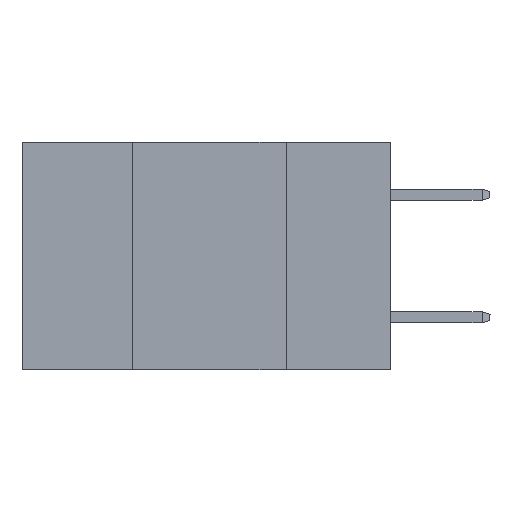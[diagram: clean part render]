
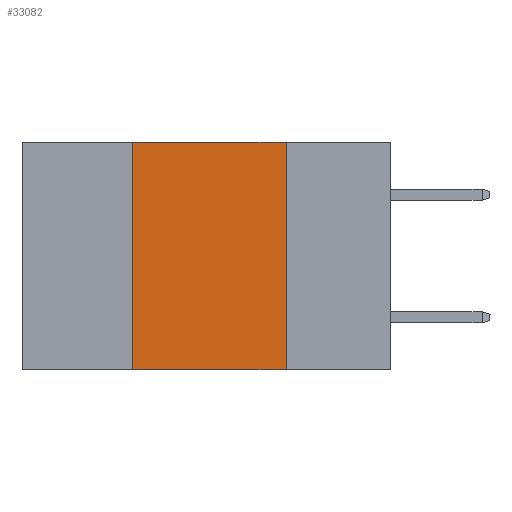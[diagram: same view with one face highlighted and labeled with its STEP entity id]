
A CAD part, left-side view. The second image highlights one B-rep face of the part: STEP entity #33082.
In plain terms, the highlighted planar face has unit normal (-1, 0, 0).
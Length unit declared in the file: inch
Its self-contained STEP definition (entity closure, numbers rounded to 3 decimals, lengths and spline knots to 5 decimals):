
#2408 = VECTOR ( 'NONE', #24869, 39.37008 ) ;
#2420 = DIRECTION ( 'NONE',  ( 0., -1., 0. ) ) ;
#3351 = LINE ( 'NONE', #26859, #30726 ) ;
#3531 = CARTESIAN_POINT ( 'NONE',  ( 0., 0.42, -0.37 ) ) ;
#4068 = ORIENTED_EDGE ( 'NONE', *, *, #39027, .F. ) ;
#4517 = VERTEX_POINT ( 'NONE', #3531 ) ;
#5360 = AXIS2_PLACEMENT_3D ( 'NONE', #18639, #31018, #36763 ) ;
#5682 = EDGE_CURVE ( 'NONE', #16432, #19999, #15143, .T. ) ;
#6515 = CARTESIAN_POINT ( 'NONE',  ( 0., 0.6, 0. ) ) ;
#6789 = CARTESIAN_POINT ( 'NONE',  ( 0., 0.17, -0.37 ) ) ;
#8766 = LINE ( 'NONE', #11761, #29892 ) ;
#8948 = VECTOR ( 'NONE', #2420, 39.37008 ) ;
#9691 = CARTESIAN_POINT ( 'NONE',  ( 0., 0.6, -0.37 ) ) ;
#10674 = ORIENTED_EDGE ( 'NONE', *, *, #31116, .F. ) ;
#11163 = ORIENTED_EDGE ( 'NONE', *, *, #38714, .T. ) ;
#11539 = DIRECTION ( 'NONE',  ( 0., 0., -1. ) ) ;
#11761 = CARTESIAN_POINT ( 'NONE',  ( 0., 0.42, 0. ) ) ;
#12148 = CARTESIAN_POINT ( 'NONE',  ( 0., 0.17, 0. ) ) ;
#12674 = FACE_OUTER_BOUND ( 'NONE', #32927, .T. ) ;
#13171 = ORIENTED_EDGE ( 'NONE', *, *, #5682, .F. ) ;
#13450 = VERTEX_POINT ( 'NONE', #6789 ) ;
#15143 = LINE ( 'NONE', #6515, #8948 ) ;
#16432 = VERTEX_POINT ( 'NONE', #28246 ) ;
#18639 = CARTESIAN_POINT ( 'NONE',  ( 0., 0.6, 0. ) ) ;
#19999 = VERTEX_POINT ( 'NONE', #12148 ) ;
#24869 = DIRECTION ( 'NONE',  ( 0., -1., 0. ) ) ;
#25961 = LINE ( 'NONE', #9691, #2408 ) ;
#26859 = CARTESIAN_POINT ( 'NONE',  ( 0., 0.17, 0. ) ) ;
#27919 = PLANE ( 'NONE',  #5360 ) ;
#28246 = CARTESIAN_POINT ( 'NONE',  ( 0., 0.42, 0. ) ) ;
#29892 = VECTOR ( 'NONE', #39467, 39.37008 ) ;
#30726 = VECTOR ( 'NONE', #11539, 39.37008 ) ;
#31018 = DIRECTION ( 'NONE',  ( 1., 0., 0. ) ) ;
#31116 = EDGE_CURVE ( 'NONE', #4517, #16432, #8766, .T. ) ;
#32927 = EDGE_LOOP ( 'NONE', ( #4068, #13171, #10674, #11163 ) ) ;
#33082 = ADVANCED_FACE ( 'NONE', ( #12674 ), #27919, .F. ) ;
#36763 = DIRECTION ( 'NONE',  ( 0., 0., -1. ) ) ;
#38714 = EDGE_CURVE ( 'NONE', #4517, #13450, #25961, .T. ) ;
#39027 = EDGE_CURVE ( 'NONE', #19999, #13450, #3351, .T. ) ;
#39467 = DIRECTION ( 'NONE',  ( 0., 0., 1. ) ) ;
